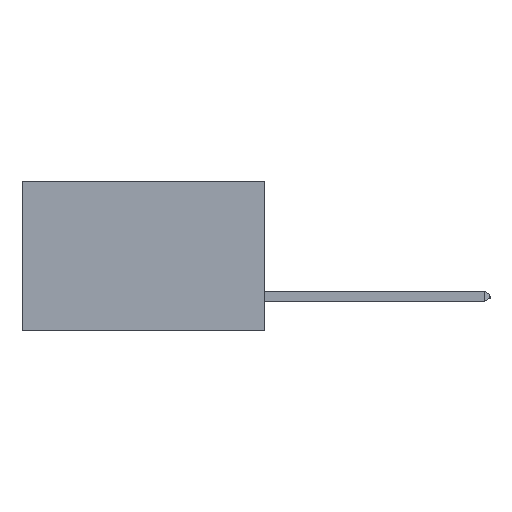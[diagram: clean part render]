
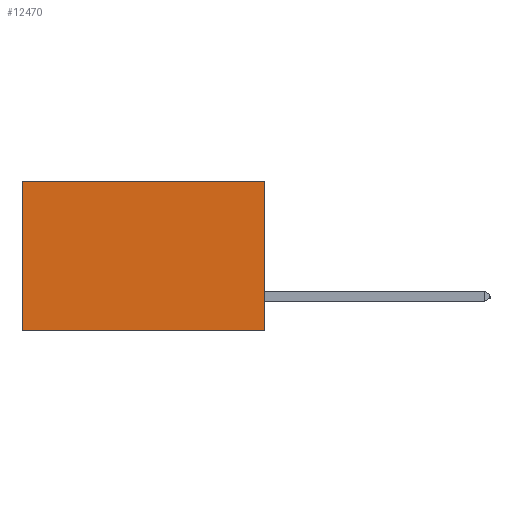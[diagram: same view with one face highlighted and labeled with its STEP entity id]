
A CAD part, left-side view. The second image highlights one B-rep face of the part: STEP entity #12470.
In plain terms, the highlighted planar face has unit normal (-1, 0, 0).
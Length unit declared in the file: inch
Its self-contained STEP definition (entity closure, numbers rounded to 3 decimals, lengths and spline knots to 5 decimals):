
#394 = VECTOR ( 'NONE', #1428, 39.37008 ) ;
#722 = EDGE_CURVE ( 'NONE', #14895, #10632, #2079, .T. ) ;
#1428 = DIRECTION ( 'NONE',  ( 0., 1., 0. ) ) ;
#2079 = LINE ( 'NONE', #15891, #10870 ) ;
#2685 = CARTESIAN_POINT ( 'NONE',  ( 0.298, 0., -0.37 ) ) ;
#3332 = ORIENTED_EDGE ( 'NONE', *, *, #722, .F. ) ;
#4260 = VERTEX_POINT ( 'NONE', #10078 ) ;
#4415 = DIRECTION ( 'NONE',  ( 0., 1., 0. ) ) ;
#4945 = ORIENTED_EDGE ( 'NONE', *, *, #16239, .T. ) ;
#5207 = ORIENTED_EDGE ( 'NONE', *, *, #14429, .T. ) ;
#5615 = ORIENTED_EDGE ( 'NONE', *, *, #19752, .F. ) ;
#7832 = VERTEX_POINT ( 'NONE', #16242 ) ;
#10078 = CARTESIAN_POINT ( 'NONE',  ( 0.298, 0.6, 0. ) ) ;
#10471 = VECTOR ( 'NONE', #18564, 39.37008 ) ;
#10632 = VERTEX_POINT ( 'NONE', #16124 ) ;
#10864 = LINE ( 'NONE', #2685, #19401 ) ;
#10870 = VECTOR ( 'NONE', #16922, 39.37008 ) ;
#11646 = EDGE_LOOP ( 'NONE', ( #4945, #5615, #3332, #5207 ) ) ;
#11699 = CARTESIAN_POINT ( 'NONE',  ( 0.298, 0.6, 0. ) ) ;
#11927 = CARTESIAN_POINT ( 'NONE',  ( 0.298, 0., 0. ) ) ;
#12470 = ADVANCED_FACE ( 'NONE', ( #20673 ), #16418, .F. ) ;
#14429 = EDGE_CURVE ( 'NONE', #14895, #4260, #18850, .T. ) ;
#14895 = VERTEX_POINT ( 'NONE', #18182 ) ;
#15085 = LINE ( 'NONE', #11699, #10471 ) ;
#15891 = CARTESIAN_POINT ( 'NONE',  ( 0.298, 0., 0. ) ) ;
#16124 = CARTESIAN_POINT ( 'NONE',  ( 0.298, 0., -0.37 ) ) ;
#16235 = DIRECTION ( 'NONE',  ( 0., 0., -1. ) ) ;
#16239 = EDGE_CURVE ( 'NONE', #4260, #7832, #15085, .T. ) ;
#16242 = CARTESIAN_POINT ( 'NONE',  ( 0.298, 0.6, -0.37 ) ) ;
#16262 = DIRECTION ( 'NONE',  ( 1., 0., 0. ) ) ;
#16418 = PLANE ( 'NONE',  #19926 ) ;
#16522 = CARTESIAN_POINT ( 'NONE',  ( 0.298, 0., 0. ) ) ;
#16922 = DIRECTION ( 'NONE',  ( 0., 0., -1. ) ) ;
#18182 = CARTESIAN_POINT ( 'NONE',  ( 0.298, 0., 0. ) ) ;
#18564 = DIRECTION ( 'NONE',  ( 0., 0., -1. ) ) ;
#18850 = LINE ( 'NONE', #11927, #394 ) ;
#19401 = VECTOR ( 'NONE', #4415, 39.37008 ) ;
#19752 = EDGE_CURVE ( 'NONE', #10632, #7832, #10864, .T. ) ;
#19926 = AXIS2_PLACEMENT_3D ( 'NONE', #16522, #16262, #16235 ) ;
#20673 = FACE_OUTER_BOUND ( 'NONE', #11646, .T. ) ;
